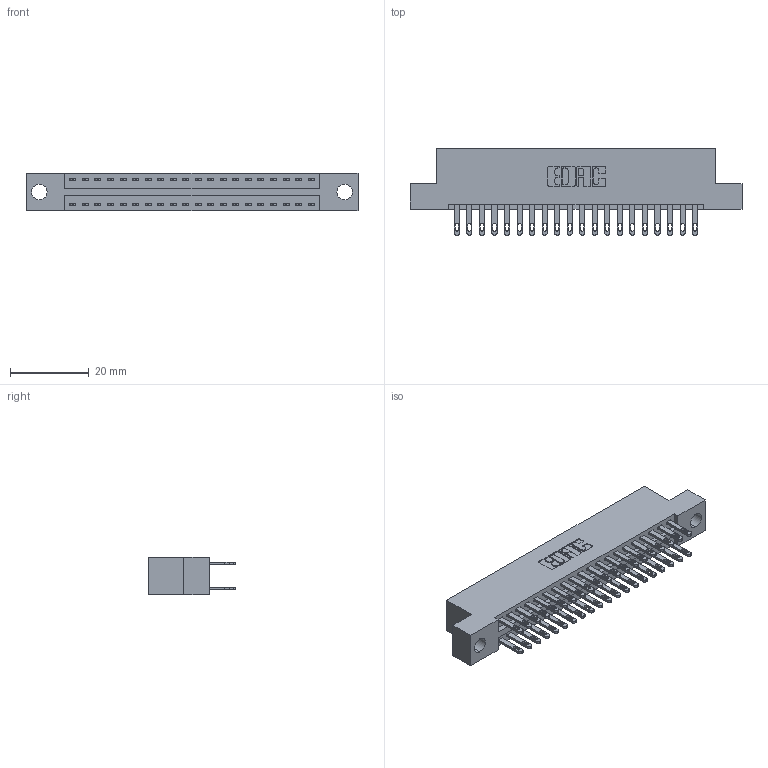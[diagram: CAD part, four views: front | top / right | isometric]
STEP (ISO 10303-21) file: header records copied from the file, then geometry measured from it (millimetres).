
FILE_DESCRIPTION (( 'STEP AP203' ), '1' );
FILE_NAME ('346-040-500-204.STEP', '2022-05-20T01:00:01', ( '' ), ( '' ), 'SwSTEP 2.0', 'SolidWorks 2020', '' );
FILE_SCHEMA (( 'CONFIG_CONTROL_DESIGN' ));
Length unit declared in the file: inch
Products named in the file (3): 345-292-001_345-293-100; 346-040-500-204; 346 Part_Flush Mounting Lugs - 0.156 Dia-TH
Assembly tree (41 placements, depth 2):
  346-040-500-204
    346 Part_Flush Mounting Lugs - 0.156 Dia-TH
    345-292-001_345-293-100  x40
Bounding box: 84.07 x 21.84 x 9.4 mm (x, y, z)
Volume: 8043.7 mm3; surface area: 10977.3 mm2
Topology: 41 solids, 41 shells, 2056 faces, 6245 edges, 4162 vertices
Faces by surface type: plane 1250, cylinder 806
Entity records: 16363 total; most frequent: CARTESIAN_POINT 2730, ORIENTED_EDGE 2662, DIRECTION 2459, EDGE_CURVE 1331, LINE 1115, VECTOR 1115, VERTEX_POINT 886, AXIS2_PLACEMENT_3D 672
